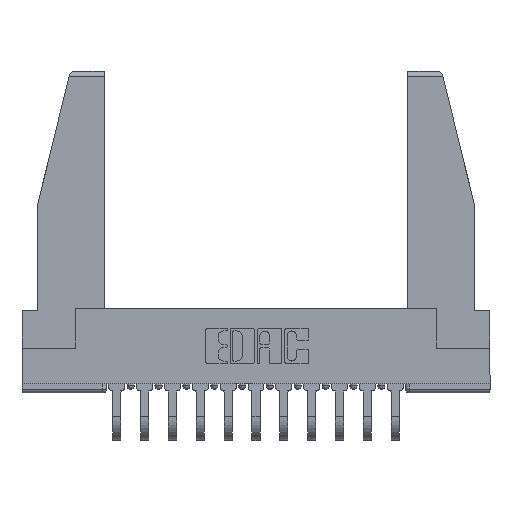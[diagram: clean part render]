
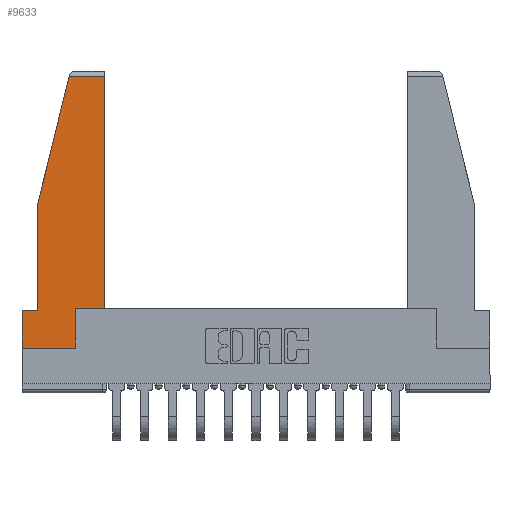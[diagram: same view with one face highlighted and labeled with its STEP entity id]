
A CAD part, top view. The second image highlights one B-rep face of the part: STEP entity #9633.
In plain terms, the highlighted planar face has unit normal (0, 0, 1).
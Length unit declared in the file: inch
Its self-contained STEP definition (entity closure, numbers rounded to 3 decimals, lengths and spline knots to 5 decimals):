
#24 = DIRECTION ( 'NONE',  ( 0., -1., 0. ) ) ;
#108 = VERTEX_POINT ( 'NONE', #12040 ) ;
#1097 = LINE ( 'NONE', #2136, #1930 ) ;
#1151 = CARTESIAN_POINT ( 'NONE',  ( 0.461, 0.223, 0. ) ) ;
#1194 = VECTOR ( 'NONE', #6698, 39.37008 ) ;
#1226 = CARTESIAN_POINT ( 'NONE',  ( 0.086, 0.8, 0. ) ) ;
#1750 = ORIENTED_EDGE ( 'NONE', *, *, #15626, .T. ) ;
#1930 = VECTOR ( 'NONE', #15663, 39.37008 ) ;
#2136 = CARTESIAN_POINT ( 'NONE',  ( 0.271, 1.55, 0. ) ) ;
#2389 = EDGE_CURVE ( 'NONE', #7726, #4694, #8554, .T. ) ;
#2473 = CARTESIAN_POINT ( 'NONE',  ( 0.297, 0., 0. ) ) ;
#3215 = CARTESIAN_POINT ( 'NONE',  ( 0.461, 0.223, 0. ) ) ;
#3319 = VECTOR ( 'NONE', #24, 39.37008 ) ;
#3361 = CARTESIAN_POINT ( 'NONE',  ( 0., 0., 0. ) ) ;
#4518 = ORIENTED_EDGE ( 'NONE', *, *, #6301, .T. ) ;
#4675 = EDGE_CURVE ( 'NONE', #6426, #9779, #9237, .T. ) ;
#4694 = VERTEX_POINT ( 'NONE', #6929 ) ;
#4699 = LINE ( 'NONE', #8692, #8875 ) ;
#5041 = EDGE_CURVE ( 'NONE', #4694, #8463, #6495, .T. ) ;
#5051 = LINE ( 'NONE', #1226, #3319 ) ;
#5151 = LINE ( 'NONE', #8913, #15320 ) ;
#5224 = VECTOR ( 'NONE', #14733, 39.37008 ) ;
#5452 = LINE ( 'NONE', #10337, #11639 ) ;
#5476 = CARTESIAN_POINT ( 'NONE',  ( 0., 0.21, 0. ) ) ;
#5608 = ORIENTED_EDGE ( 'NONE', *, *, #4675, .T. ) ;
#5643 = ORIENTED_EDGE ( 'NONE', *, *, #8541, .T. ) ;
#6004 = CARTESIAN_POINT ( 'NONE',  ( 0.086, 0.21, 0. ) ) ;
#6301 = EDGE_CURVE ( 'NONE', #12525, #6426, #4699, .T. ) ;
#6426 = VERTEX_POINT ( 'NONE', #12136 ) ;
#6495 = LINE ( 'NONE', #7041, #12984 ) ;
#6698 = DIRECTION ( 'NONE',  ( 0., 1., 0. ) ) ;
#6929 = CARTESIAN_POINT ( 'NONE',  ( 0.297, 0.223, 0. ) ) ;
#7041 = CARTESIAN_POINT ( 'NONE',  ( 0.297, 0.223, 0. ) ) ;
#7266 = EDGE_LOOP ( 'NONE', ( #14461, #1750, #13692, #5643, #4518, #5608, #13618, #10770, #12448 ) ) ;
#7695 = PLANE ( 'NONE',  #13160 ) ;
#7726 = VERTEX_POINT ( 'NONE', #9595 ) ;
#8431 = LINE ( 'NONE', #1151, #1194 ) ;
#8463 = VERTEX_POINT ( 'NONE', #3215 ) ;
#8541 = EDGE_CURVE ( 'NONE', #108, #12525, #5051, .T. ) ;
#8554 = LINE ( 'NONE', #2473, #5224 ) ;
#8692 = CARTESIAN_POINT ( 'NONE',  ( 0., 0.21, 0. ) ) ;
#8875 = VECTOR ( 'NONE', #9979, 39.37008 ) ;
#8913 = CARTESIAN_POINT ( 'NONE',  ( 0., 1.52, 0. ) ) ;
#9237 = LINE ( 'NONE', #5476, #15539 ) ;
#9595 = CARTESIAN_POINT ( 'NONE',  ( 0.297, 0., 0. ) ) ;
#9633 = ADVANCED_FACE ( 'NONE', ( #10090 ), #7695, .T. ) ;
#9779 = VERTEX_POINT ( 'NONE', #3361 ) ;
#9979 = DIRECTION ( 'NONE',  ( -1., 0., 0. ) ) ;
#10090 = FACE_OUTER_BOUND ( 'NONE', #7266, .T. ) ;
#10146 = EDGE_CURVE ( 'NONE', #12281, #108, #1097, .T. ) ;
#10337 = CARTESIAN_POINT ( 'NONE',  ( 0., 0., 0. ) ) ;
#10770 = ORIENTED_EDGE ( 'NONE', *, *, #2389, .T. ) ;
#10980 = EDGE_CURVE ( 'NONE', #9779, #7726, #5452, .T. ) ;
#11372 = DIRECTION ( 'NONE',  ( 1., 0., 0. ) ) ;
#11639 = VECTOR ( 'NONE', #15221, 39.37008 ) ;
#11926 = DIRECTION ( 'NONE',  ( 1., 0., 0. ) ) ;
#11981 = EDGE_CURVE ( 'NONE', #8463, #12298, #8431, .T. ) ;
#12040 = CARTESIAN_POINT ( 'NONE',  ( 0.086, 0.8, 0. ) ) ;
#12136 = CARTESIAN_POINT ( 'NONE',  ( 0., 0.21, 0. ) ) ;
#12281 = VERTEX_POINT ( 'NONE', #12659 ) ;
#12298 = VERTEX_POINT ( 'NONE', #15149 ) ;
#12448 = ORIENTED_EDGE ( 'NONE', *, *, #5041, .T. ) ;
#12525 = VERTEX_POINT ( 'NONE', #6004 ) ;
#12579 = DIRECTION ( 'NONE',  ( 0., 0., 1. ) ) ;
#12651 = CARTESIAN_POINT ( 'NONE',  ( 0., 0., 0. ) ) ;
#12659 = CARTESIAN_POINT ( 'NONE',  ( 0.2636, 1.52, 0. ) ) ;
#12984 = VECTOR ( 'NONE', #11926, 39.37008 ) ;
#13160 = AXIS2_PLACEMENT_3D ( 'NONE', #12651, #12579, #11372 ) ;
#13618 = ORIENTED_EDGE ( 'NONE', *, *, #10980, .T. ) ;
#13692 = ORIENTED_EDGE ( 'NONE', *, *, #10146, .T. ) ;
#13960 = DIRECTION ( 'NONE',  ( -1., 0., 0. ) ) ;
#14461 = ORIENTED_EDGE ( 'NONE', *, *, #11981, .T. ) ;
#14733 = DIRECTION ( 'NONE',  ( 0., 1., 0. ) ) ;
#15149 = CARTESIAN_POINT ( 'NONE',  ( 0.461, 1.52, 0. ) ) ;
#15221 = DIRECTION ( 'NONE',  ( 1., 0., 0. ) ) ;
#15320 = VECTOR ( 'NONE', #13960, 39.37008 ) ;
#15410 = DIRECTION ( 'NONE',  ( 0., -1., 0. ) ) ;
#15539 = VECTOR ( 'NONE', #15410, 39.37008 ) ;
#15626 = EDGE_CURVE ( 'NONE', #12298, #12281, #5151, .T. ) ;
#15663 = DIRECTION ( 'NONE',  ( -0.239, -0.971, 0. ) ) ;
